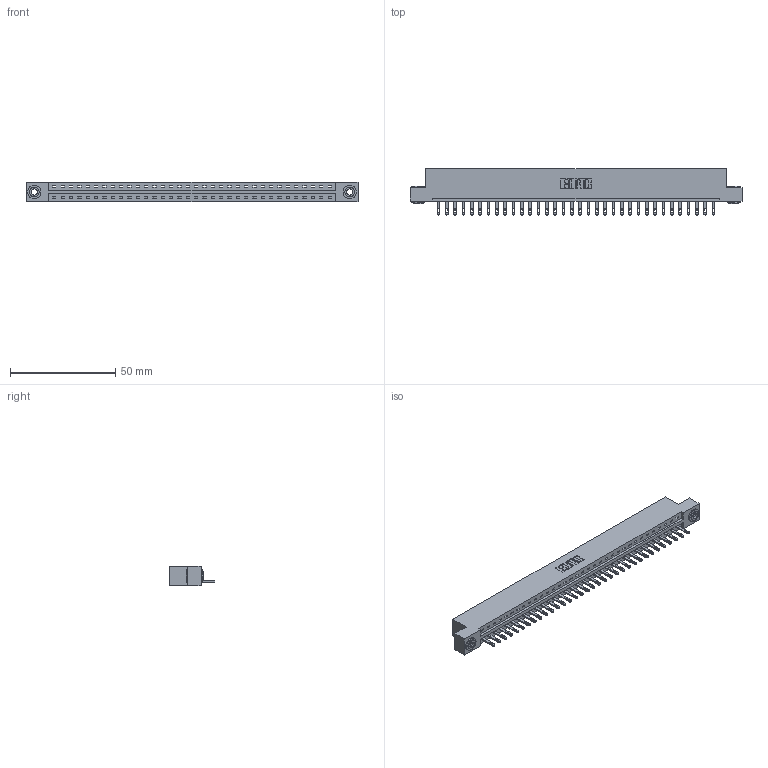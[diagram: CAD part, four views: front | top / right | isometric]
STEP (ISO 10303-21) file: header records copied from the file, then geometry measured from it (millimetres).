
FILE_DESCRIPTION (( 'STEP AP203' ), '1' );
FILE_NAME ('887-034-500-103.STEP', '2020-09-20T21:33:40', ( '' ), ( '' ), 'SwSTEP 2.0', 'SolidWorks 2020', '' );
FILE_SCHEMA (( 'CONFIG_CONTROL_DESIGN' ));
Length unit declared in the file: inch
Products named in the file (4): 837 Part_Flush Mounting Lugs - 0.156 Dia-TH; 887-034-500-103; 345-292-001_345-293-100; 345-250-002_345-250-002-102
Assembly tree (37 placements, depth 2):
  887-034-500-103
    837 Part_Flush Mounting Lugs - 0.156 Dia-TH
    345-292-001_345-293-100  x34
    345-250-002_345-250-002-102  x2
Bounding box: 157.73 x 21.85 x 9.4 mm (x, y, z)
Volume: 16334.1 mm3; surface area: 17146.6 mm2
Topology: 37 solids, 37 shells, 2124 faces, 6507 edges, 4334 vertices
Faces by surface type: plane 1440, cylinder 676, cone 8
Entity records: 26888 total; most frequent: CARTESIAN_POINT 4659, ORIENTED_EDGE 4622, DIRECTION 3973, EDGE_CURVE 2311, VECTOR 2155, LINE 2155, VERTEX_POINT 1538, AXIS2_PLACEMENT_3D 909
